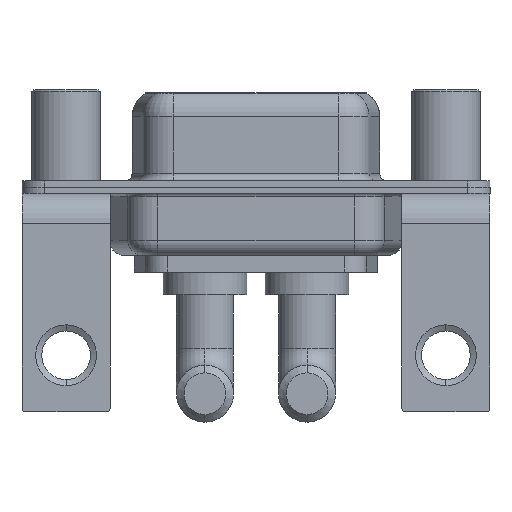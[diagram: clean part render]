
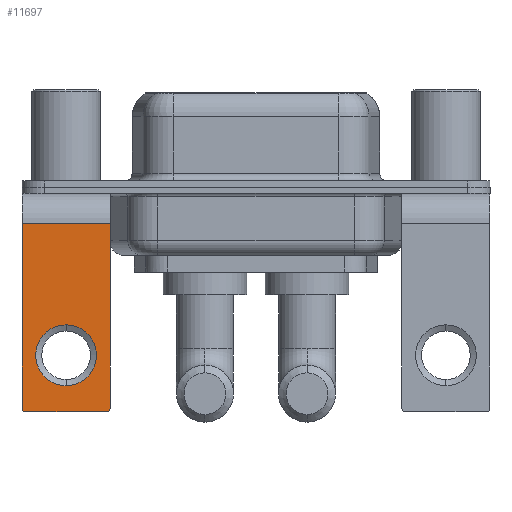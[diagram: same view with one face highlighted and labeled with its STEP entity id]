
A CAD part, front view. The second image highlights one B-rep face of the part: STEP entity #11697.
In plain terms, the highlighted planar face has unit normal (0, -1, 0).
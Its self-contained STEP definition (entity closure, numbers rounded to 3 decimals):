
#113 = AXIS2_PLACEMENT_3D ( 'NONE', #9174, #2118, #13636 ) ;
#185 = EDGE_CURVE ( 'NONE', #8896, #10694, #3750, .T. ) ;
#255 = DIRECTION ( 'NONE',  ( 0., 0., 1. ) ) ;
#336 = VECTOR ( 'NONE', #4373, 1000. ) ;
#737 = VERTEX_POINT ( 'NONE', #4915 ) ;
#1079 = FACE_OUTER_BOUND ( 'NONE', #10762, .T. ) ;
#1210 = VERTEX_POINT ( 'NONE', #6959 ) ;
#2118 = DIRECTION ( 'NONE',  ( 0., 1., 0. ) ) ;
#2409 = CARTESIAN_POINT ( 'NONE',  ( -2.9, -6.25, -2.4 ) ) ;
#2782 = CIRCLE ( 'NONE', #7546, 0.25 ) ;
#2810 = CARTESIAN_POINT ( 'NONE',  ( 2.9, -6.25, -2.4 ) ) ;
#2952 = DIRECTION ( 'NONE',  ( -1., 0., 0. ) ) ;
#3032 = DIRECTION ( 'NONE',  ( 0., -1., 0. ) ) ;
#3437 = EDGE_CURVE ( 'NONE', #10694, #8896, #6866, .T. ) ;
#3499 = AXIS2_PLACEMENT_3D ( 'NONE', #12235, #11192, #9242 ) ;
#3539 = EDGE_CURVE ( 'NONE', #1210, #8324, #8770, .T. ) ;
#3750 = CIRCLE ( 'NONE', #3499, 2. ) ;
#4082 = CARTESIAN_POINT ( 'NONE',  ( 0., -6.25, -9.07 ) ) ;
#4373 = DIRECTION ( 'NONE',  ( 0., 0., -1. ) ) ;
#4589 = VECTOR ( 'NONE', #12122, 1000. ) ;
#4915 = CARTESIAN_POINT ( 'NONE',  ( 2.9, -6.25, -2.4 ) ) ;
#4978 = AXIS2_PLACEMENT_3D ( 'NONE', #11688, #5889, #255 ) ;
#5185 = EDGE_CURVE ( 'NONE', #6065, #6828, #2782, .T. ) ;
#5749 = PLANE ( 'NONE',  #113 ) ;
#5889 = DIRECTION ( 'NONE',  ( 0., 1., 0. ) ) ;
#6065 = VERTEX_POINT ( 'NONE', #7607 ) ;
#6292 = ORIENTED_EDGE ( 'NONE', *, *, #14505, .T. ) ;
#6520 = CARTESIAN_POINT ( 'NONE',  ( 2.65, -6.25, -14.55 ) ) ;
#6589 = CARTESIAN_POINT ( 'NONE',  ( 2.9, -6.25, -2.4 ) ) ;
#6644 = AXIS2_PLACEMENT_3D ( 'NONE', #12346, #13674, #12410 ) ;
#6787 = FACE_BOUND ( 'NONE', #12961, .T. ) ;
#6828 = VERTEX_POINT ( 'NONE', #7251 ) ;
#6866 = CIRCLE ( 'NONE', #4978, 2. ) ;
#6959 = CARTESIAN_POINT ( 'NONE',  ( -2.9, -6.25, -14.55 ) ) ;
#7012 = VECTOR ( 'NONE', #2952, 1000. ) ;
#7251 = CARTESIAN_POINT ( 'NONE',  ( 2.9, -6.25, -14.55 ) ) ;
#7546 = AXIS2_PLACEMENT_3D ( 'NONE', #6520, #3032, #9930 ) ;
#7562 = ORIENTED_EDGE ( 'NONE', *, *, #185, .T. ) ;
#7607 = CARTESIAN_POINT ( 'NONE',  ( 2.65, -6.25, -14.8 ) ) ;
#7612 = ORIENTED_EDGE ( 'NONE', *, *, #5185, .T. ) ;
#8279 = CARTESIAN_POINT ( 'NONE',  ( -2.65, -6.25, -14.8 ) ) ;
#8324 = VERTEX_POINT ( 'NONE', #8279 ) ;
#8509 = EDGE_CURVE ( 'NONE', #6065, #8324, #8856, .T. ) ;
#8661 = ORIENTED_EDGE ( 'NONE', *, *, #10934, .F. ) ;
#8770 = CIRCLE ( 'NONE', #6644, 0.25 ) ;
#8856 = LINE ( 'NONE', #11970, #4589 ) ;
#8896 = VERTEX_POINT ( 'NONE', #4082 ) ;
#9174 = CARTESIAN_POINT ( 'NONE',  ( 2.9, -6.25, -2.4 ) ) ;
#9242 = DIRECTION ( 'NONE',  ( 0., 0., 1. ) ) ;
#9576 = ORIENTED_EDGE ( 'NONE', *, *, #3539, .T. ) ;
#9788 = ORIENTED_EDGE ( 'NONE', *, *, #8509, .F. ) ;
#9930 = DIRECTION ( 'NONE',  ( 0., 0., 1. ) ) ;
#10694 = VERTEX_POINT ( 'NONE', #14247 ) ;
#10762 = EDGE_LOOP ( 'NONE', ( #6292, #9576, #9788, #7612, #8661, #13962 ) ) ;
#10833 = DIRECTION ( 'NONE',  ( 0., 0., -1. ) ) ;
#10934 = EDGE_CURVE ( 'NONE', #737, #6828, #14547, .T. ) ;
#11078 = VECTOR ( 'NONE', #10833, 1000. ) ;
#11192 = DIRECTION ( 'NONE',  ( 0., 1., 0. ) ) ;
#11688 = CARTESIAN_POINT ( 'NONE',  ( 0., -6.25, -11.07 ) ) ;
#11697 = ADVANCED_FACE ( 'NONE', ( #6787, #1079 ), #5749, .F. ) ;
#11970 = CARTESIAN_POINT ( 'NONE',  ( 2.9, -6.25, -14.8 ) ) ;
#12004 = ORIENTED_EDGE ( 'NONE', *, *, #3437, .T. ) ;
#12006 = VERTEX_POINT ( 'NONE', #2409 ) ;
#12122 = DIRECTION ( 'NONE',  ( -1., 0., 0. ) ) ;
#12235 = CARTESIAN_POINT ( 'NONE',  ( 0., -6.25, -11.07 ) ) ;
#12346 = CARTESIAN_POINT ( 'NONE',  ( -2.65, -6.25, -14.55 ) ) ;
#12410 = DIRECTION ( 'NONE',  ( 0., 0., 1. ) ) ;
#12961 = EDGE_LOOP ( 'NONE', ( #12004, #7562 ) ) ;
#12989 = LINE ( 'NONE', #2810, #7012 ) ;
#13141 = CARTESIAN_POINT ( 'NONE',  ( -2.9, -6.25, -2.4 ) ) ;
#13189 = EDGE_CURVE ( 'NONE', #737, #12006, #12989, .T. ) ;
#13636 = DIRECTION ( 'NONE',  ( 0., 0., 1. ) ) ;
#13674 = DIRECTION ( 'NONE',  ( 0., -1., 0. ) ) ;
#13962 = ORIENTED_EDGE ( 'NONE', *, *, #13189, .T. ) ;
#14247 = CARTESIAN_POINT ( 'NONE',  ( 0., -6.25, -13.07 ) ) ;
#14330 = LINE ( 'NONE', #13141, #11078 ) ;
#14505 = EDGE_CURVE ( 'NONE', #12006, #1210, #14330, .T. ) ;
#14547 = LINE ( 'NONE', #6589, #336 ) ;
